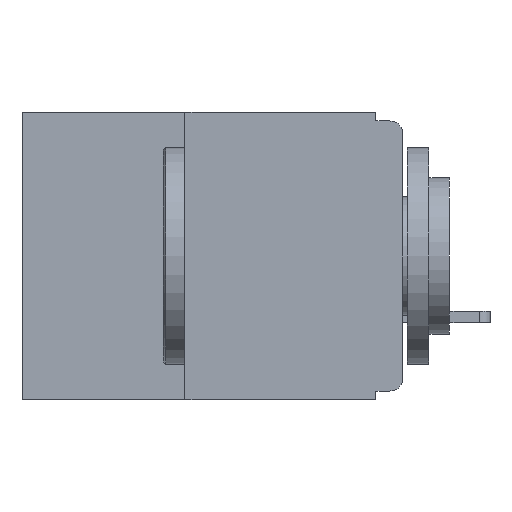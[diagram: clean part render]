
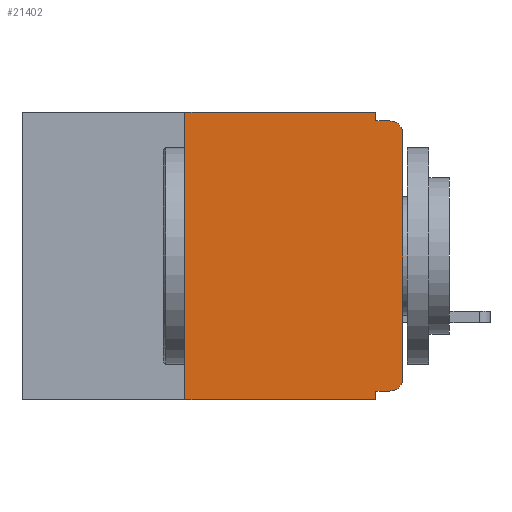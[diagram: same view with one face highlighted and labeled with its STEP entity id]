
A CAD part, left-side view. The second image highlights one B-rep face of the part: STEP entity #21402.
In plain terms, the highlighted planar face has unit normal (-1, 0, 0).
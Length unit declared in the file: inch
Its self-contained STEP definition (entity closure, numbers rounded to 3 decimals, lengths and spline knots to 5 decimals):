
#303 = EDGE_LOOP ( 'NONE', ( #29440, #22200, #14107, #13298, #9606, #23113, #11318, #18929, #15683, #22612 ) ) ;
#769 = VERTEX_POINT ( 'NONE', #21374 ) ;
#886 = DIRECTION ( 'NONE',  ( 0., -1., 0. ) ) ;
#977 = EDGE_CURVE ( 'NONE', #769, #6153, #8222, .T. ) ;
#1254 = DIRECTION ( 'NONE',  ( 0., 0., -1. ) ) ;
#1256 = CARTESIAN_POINT ( 'NONE',  ( 0., 0.25, -0.33 ) ) ;
#1289 = LINE ( 'NONE', #5171, #28228 ) ;
#3910 = CARTESIAN_POINT ( 'NONE',  ( 0., 0.031, 0. ) ) ;
#4107 = AXIS2_PLACEMENT_3D ( 'NONE', #32313, #32132, #7105 ) ;
#4609 = EDGE_CURVE ( 'NONE', #14020, #9865, #4671, .T. ) ;
#4613 = CARTESIAN_POINT ( 'NONE',  ( 0., 0.015, -0.025 ) ) ;
#4671 = LINE ( 'NONE', #25241, #10848 ) ;
#5041 = CARTESIAN_POINT ( 'NONE',  ( 0., 0.25, -0.33 ) ) ;
#5171 = CARTESIAN_POINT ( 'NONE',  ( 0., 0.437, -0.33 ) ) ;
#5331 = VERTEX_POINT ( 'NONE', #17951 ) ;
#5749 = CARTESIAN_POINT ( 'NONE',  ( 0., 0., 0. ) ) ;
#5896 = FACE_OUTER_BOUND ( 'NONE', #303, .T. ) ;
#6153 = VERTEX_POINT ( 'NONE', #13597 ) ;
#6724 = EDGE_CURVE ( 'NONE', #32565, #5331, #30011, .T. ) ;
#7105 = DIRECTION ( 'NONE',  ( 0., 0., -1. ) ) ;
#7271 = DIRECTION ( 'NONE',  ( 0., 0., -1. ) ) ;
#8077 = VERTEX_POINT ( 'NONE', #10523 ) ;
#8222 = CIRCLE ( 'NONE', #4107, 0.015 ) ;
#8522 = DIRECTION ( 'NONE',  ( 0., 1., 0. ) ) ;
#8851 = EDGE_CURVE ( 'NONE', #769, #25026, #12374, .T. ) ;
#9069 = DIRECTION ( 'NONE',  ( 0., 0., -1. ) ) ;
#9606 = ORIENTED_EDGE ( 'NONE', *, *, #4609, .F. ) ;
#9865 = VERTEX_POINT ( 'NONE', #16108 ) ;
#10523 = CARTESIAN_POINT ( 'NONE',  ( 0., 0.031, -0.01 ) ) ;
#10848 = VECTOR ( 'NONE', #12187, 39.37008 ) ;
#11318 = ORIENTED_EDGE ( 'NONE', *, *, #29456, .T. ) ;
#12187 = DIRECTION ( 'NONE',  ( 0., -1., 0. ) ) ;
#12374 = LINE ( 'NONE', #29208, #32246 ) ;
#12631 = CARTESIAN_POINT ( 'NONE',  ( 0., 0.031, -0.32 ) ) ;
#12816 = VECTOR ( 'NONE', #886, 39.37008 ) ;
#13298 = ORIENTED_EDGE ( 'NONE', *, *, #24814, .F. ) ;
#13597 = CARTESIAN_POINT ( 'NONE',  ( 0., 0., -0.305 ) ) ;
#13672 = EDGE_CURVE ( 'NONE', #6153, #32565, #19414, .T. ) ;
#14020 = VERTEX_POINT ( 'NONE', #17855 ) ;
#14107 = ORIENTED_EDGE ( 'NONE', *, *, #17206, .F. ) ;
#14252 = CARTESIAN_POINT ( 'NONE',  ( 0., 0.437, 0. ) ) ;
#15683 = ORIENTED_EDGE ( 'NONE', *, *, #8851, .F. ) ;
#16108 = CARTESIAN_POINT ( 'NONE',  ( 0., 0.031, 0. ) ) ;
#16119 = LINE ( 'NONE', #32749, #21436 ) ;
#16718 = EDGE_CURVE ( 'NONE', #25026, #18181, #16119, .T. ) ;
#17206 = EDGE_CURVE ( 'NONE', #8077, #5331, #19760, .T. ) ;
#17266 = EDGE_CURVE ( 'NONE', #20128, #14020, #30261, .T. ) ;
#17855 = CARTESIAN_POINT ( 'NONE',  ( 0., 0.25, 0. ) ) ;
#17951 = CARTESIAN_POINT ( 'NONE',  ( 0., 0.015, -0.01 ) ) ;
#18181 = VERTEX_POINT ( 'NONE', #20413 ) ;
#18929 = ORIENTED_EDGE ( 'NONE', *, *, #16718, .F. ) ;
#19414 = LINE ( 'NONE', #5749, #25477 ) ;
#19760 = LINE ( 'NONE', #32144, #12816 ) ;
#19763 = DIRECTION ( 'NONE',  ( 0., 0., -1. ) ) ;
#20128 = VERTEX_POINT ( 'NONE', #5041 ) ;
#20373 = AXIS2_PLACEMENT_3D ( 'NONE', #4613, #22908, #7271 ) ;
#20413 = CARTESIAN_POINT ( 'NONE',  ( 0., 0.031, -0.33 ) ) ;
#20990 = DIRECTION ( 'NONE',  ( 0., -1., 0. ) ) ;
#21374 = CARTESIAN_POINT ( 'NONE',  ( 0., 0.015, -0.32 ) ) ;
#21402 = ADVANCED_FACE ( 'NONE', ( #5896 ), #32352, .F. ) ;
#21436 = VECTOR ( 'NONE', #19763, 39.37008 ) ;
#22200 = ORIENTED_EDGE ( 'NONE', *, *, #6724, .T. ) ;
#22612 = ORIENTED_EDGE ( 'NONE', *, *, #977, .T. ) ;
#22908 = DIRECTION ( 'NONE',  ( -1., 0., 0. ) ) ;
#23113 = ORIENTED_EDGE ( 'NONE', *, *, #17266, .F. ) ;
#23374 = VECTOR ( 'NONE', #24793, 39.37008 ) ;
#24000 = DIRECTION ( 'NONE',  ( 0., 0., 1. ) ) ;
#24480 = VECTOR ( 'NONE', #1254, 39.37008 ) ;
#24677 = DIRECTION ( 'NONE',  ( 1., 0., 0. ) ) ;
#24793 = DIRECTION ( 'NONE',  ( 0., 0., 1. ) ) ;
#24814 = EDGE_CURVE ( 'NONE', #9865, #8077, #25283, .T. ) ;
#25026 = VERTEX_POINT ( 'NONE', #12631 ) ;
#25241 = CARTESIAN_POINT ( 'NONE',  ( 0., 0.437, 0. ) ) ;
#25283 = LINE ( 'NONE', #3910, #24480 ) ;
#25477 = VECTOR ( 'NONE', #24000, 39.37008 ) ;
#27016 = AXIS2_PLACEMENT_3D ( 'NONE', #14252, #24677, #9069 ) ;
#28228 = VECTOR ( 'NONE', #20990, 39.37008 ) ;
#29208 = CARTESIAN_POINT ( 'NONE',  ( 0., 0., -0.32 ) ) ;
#29440 = ORIENTED_EDGE ( 'NONE', *, *, #13672, .T. ) ;
#29456 = EDGE_CURVE ( 'NONE', #20128, #18181, #1289, .T. ) ;
#30011 = CIRCLE ( 'NONE', #20373, 0.015 ) ;
#30261 = LINE ( 'NONE', #1256, #23374 ) ;
#31442 = CARTESIAN_POINT ( 'NONE',  ( 0., 0., -0.025 ) ) ;
#32132 = DIRECTION ( 'NONE',  ( -1., 0., 0. ) ) ;
#32144 = CARTESIAN_POINT ( 'NONE',  ( 0., 0., -0.01 ) ) ;
#32246 = VECTOR ( 'NONE', #8522, 39.37008 ) ;
#32313 = CARTESIAN_POINT ( 'NONE',  ( 0., 0.015, -0.305 ) ) ;
#32352 = PLANE ( 'NONE',  #27016 ) ;
#32565 = VERTEX_POINT ( 'NONE', #31442 ) ;
#32749 = CARTESIAN_POINT ( 'NONE',  ( 0., 0.031, -0.33 ) ) ;
